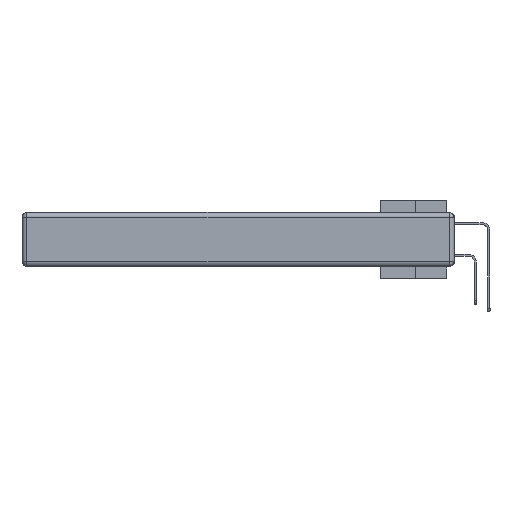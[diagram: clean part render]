
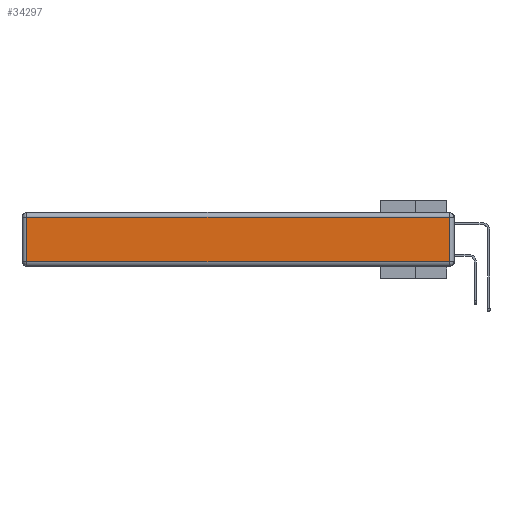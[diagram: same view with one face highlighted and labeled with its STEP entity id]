
A CAD part, left-side view. The second image highlights one B-rep face of the part: STEP entity #34297.
In plain terms, the highlighted planar face has unit normal (-1, 0, 0).
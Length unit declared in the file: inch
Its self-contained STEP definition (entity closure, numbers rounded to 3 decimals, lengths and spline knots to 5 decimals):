
#2251 = VERTEX_POINT ( 'NONE', #17531 ) ;
#3011 = EDGE_CURVE ( 'NONE', #37612, #7701, #26301, .T. ) ;
#3998 = CARTESIAN_POINT ( 'NONE',  ( 0., 0.03, -0.313 ) ) ;
#5208 = EDGE_LOOP ( 'NONE', ( #29998, #25539, #19812, #16764 ) ) ;
#6558 = DIRECTION ( 'NONE',  ( -1., 0., 0. ) ) ;
#7701 = VERTEX_POINT ( 'NONE', #19680 ) ;
#8864 = VECTOR ( 'NONE', #17598, 39.37008 ) ;
#12658 = EDGE_CURVE ( 'NONE', #2251, #37612, #26147, .T. ) ;
#12835 = CARTESIAN_POINT ( 'NONE',  ( 0., 0., -0.343 ) ) ;
#14701 = VECTOR ( 'NONE', #23787, 39.37008 ) ;
#16382 = CARTESIAN_POINT ( 'NONE',  ( 0., 2.72, -0.343 ) ) ;
#16420 = DIRECTION ( 'NONE',  ( 0., 1., 0. ) ) ;
#16764 = ORIENTED_EDGE ( 'NONE', *, *, #3011, .T. ) ;
#17510 = LINE ( 'NONE', #23584, #14701 ) ;
#17531 = CARTESIAN_POINT ( 'NONE',  ( 0., 0.03, -0.03 ) ) ;
#17598 = DIRECTION ( 'NONE',  ( 0., 0., 1. ) ) ;
#19121 = EDGE_CURVE ( 'NONE', #34790, #2251, #26109, .T. ) ;
#19538 = VECTOR ( 'NONE', #16420, 39.37008 ) ;
#19680 = CARTESIAN_POINT ( 'NONE',  ( 0., 2.72, -0.313 ) ) ;
#19812 = ORIENTED_EDGE ( 'NONE', *, *, #12658, .T. ) ;
#21968 = PLANE ( 'NONE',  #28125 ) ;
#22173 = FACE_OUTER_BOUND ( 'NONE', #5208, .T. ) ;
#23258 = CARTESIAN_POINT ( 'NONE',  ( 0., 0.03, -0.343 ) ) ;
#23584 = CARTESIAN_POINT ( 'NONE',  ( 0., 0., -0.313 ) ) ;
#23787 = DIRECTION ( 'NONE',  ( 0., -1., 0. ) ) ;
#25539 = ORIENTED_EDGE ( 'NONE', *, *, #19121, .T. ) ;
#26109 = LINE ( 'NONE', #23258, #8864 ) ;
#26147 = LINE ( 'NONE', #38309, #19538 ) ;
#26301 = LINE ( 'NONE', #16382, #30292 ) ;
#28064 = DIRECTION ( 'NONE',  ( 0., 0., 1. ) ) ;
#28125 = AXIS2_PLACEMENT_3D ( 'NONE', #12835, #6558, #28064 ) ;
#28430 = CARTESIAN_POINT ( 'NONE',  ( 0., 2.72, -0.03 ) ) ;
#28953 = DIRECTION ( 'NONE',  ( 0., 0., -1. ) ) ;
#29998 = ORIENTED_EDGE ( 'NONE', *, *, #37250, .T. ) ;
#30292 = VECTOR ( 'NONE', #28953, 39.37008 ) ;
#34297 = ADVANCED_FACE ( 'NONE', ( #22173 ), #21968, .T. ) ;
#34790 = VERTEX_POINT ( 'NONE', #3998 ) ;
#37250 = EDGE_CURVE ( 'NONE', #7701, #34790, #17510, .T. ) ;
#37612 = VERTEX_POINT ( 'NONE', #28430 ) ;
#38309 = CARTESIAN_POINT ( 'NONE',  ( 0., 2.75, -0.03 ) ) ;
